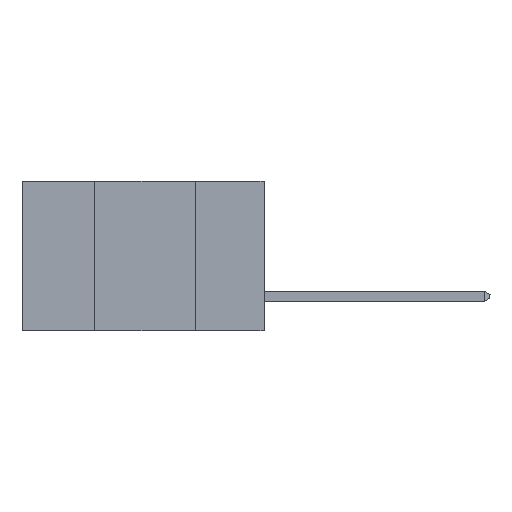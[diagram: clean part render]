
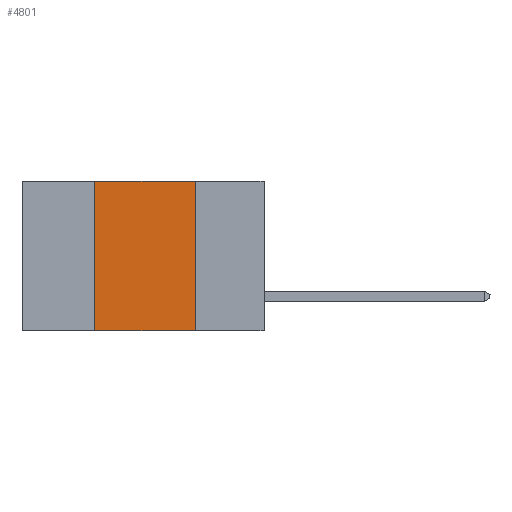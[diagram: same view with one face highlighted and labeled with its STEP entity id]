
A CAD part, left-side view. The second image highlights one B-rep face of the part: STEP entity #4801.
In plain terms, the highlighted planar face has unit normal (-1, 0, 0).
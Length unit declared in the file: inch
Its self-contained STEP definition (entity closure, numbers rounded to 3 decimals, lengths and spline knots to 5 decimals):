
#482 = CARTESIAN_POINT ( 'NONE',  ( 0., 0.17, 0. ) ) ;
#1040 = PLANE ( 'NONE',  #4558 ) ;
#2030 = CARTESIAN_POINT ( 'NONE',  ( 0., 0.42, -0.37 ) ) ;
#2258 = EDGE_CURVE ( 'NONE', #2553, #3603, #8906, .T. ) ;
#2352 = CARTESIAN_POINT ( 'NONE',  ( 0., 0.17, 0. ) ) ;
#2473 = CARTESIAN_POINT ( 'NONE',  ( 0., 0.42, 0. ) ) ;
#2525 = VERTEX_POINT ( 'NONE', #2473 ) ;
#2553 = VERTEX_POINT ( 'NONE', #482 ) ;
#3211 = DIRECTION ( 'NONE',  ( 0., 0., -1. ) ) ;
#3603 = VERTEX_POINT ( 'NONE', #4043 ) ;
#3706 = LINE ( 'NONE', #7571, #8864 ) ;
#3873 = FACE_OUTER_BOUND ( 'NONE', #6338, .T. ) ;
#4043 = CARTESIAN_POINT ( 'NONE',  ( 0., 0.17, -0.37 ) ) ;
#4074 = DIRECTION ( 'NONE',  ( 0., -1., 0. ) ) ;
#4409 = ORIENTED_EDGE ( 'NONE', *, *, #7457, .T. ) ;
#4558 = AXIS2_PLACEMENT_3D ( 'NONE', #6754, #7486, #3211 ) ;
#4624 = EDGE_CURVE ( 'NONE', #8234, #2525, #6758, .T. ) ;
#4801 = ADVANCED_FACE ( 'NONE', ( #3873 ), #1040, .F. ) ;
#4859 = VECTOR ( 'NONE', #5449, 39.37008 ) ;
#5142 = CARTESIAN_POINT ( 'NONE',  ( 0., 0.42, 0. ) ) ;
#5189 = VECTOR ( 'NONE', #7417, 39.37008 ) ;
#5449 = DIRECTION ( 'NONE',  ( 0., -1., 0. ) ) ;
#6338 = EDGE_LOOP ( 'NONE', ( #6861, #7443, #6816, #4409 ) ) ;
#6754 = CARTESIAN_POINT ( 'NONE',  ( 0., 0.6, 0. ) ) ;
#6758 = LINE ( 'NONE', #5142, #8110 ) ;
#6770 = LINE ( 'NONE', #6830, #4859 ) ;
#6816 = ORIENTED_EDGE ( 'NONE', *, *, #4624, .F. ) ;
#6830 = CARTESIAN_POINT ( 'NONE',  ( 0., 0.6, -0.37 ) ) ;
#6861 = ORIENTED_EDGE ( 'NONE', *, *, #2258, .F. ) ;
#7326 = DIRECTION ( 'NONE',  ( 0., 0., 1. ) ) ;
#7417 = DIRECTION ( 'NONE',  ( 0., 0., -1. ) ) ;
#7443 = ORIENTED_EDGE ( 'NONE', *, *, #9139, .F. ) ;
#7457 = EDGE_CURVE ( 'NONE', #8234, #3603, #6770, .T. ) ;
#7486 = DIRECTION ( 'NONE',  ( 1., 0., 0. ) ) ;
#7571 = CARTESIAN_POINT ( 'NONE',  ( 0., 0.6, 0. ) ) ;
#8110 = VECTOR ( 'NONE', #7326, 39.37008 ) ;
#8234 = VERTEX_POINT ( 'NONE', #2030 ) ;
#8864 = VECTOR ( 'NONE', #4074, 39.37008 ) ;
#8906 = LINE ( 'NONE', #2352, #5189 ) ;
#9139 = EDGE_CURVE ( 'NONE', #2525, #2553, #3706, .T. ) ;
